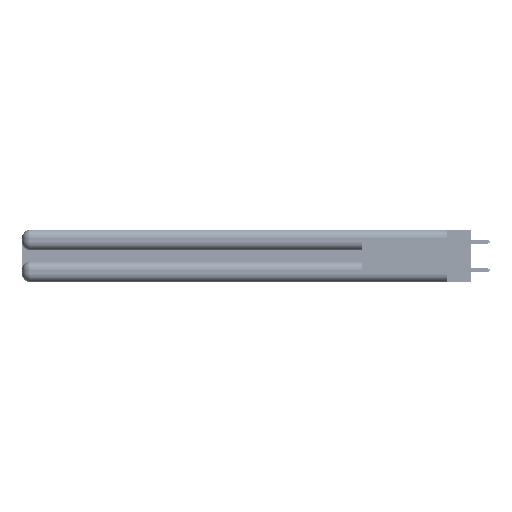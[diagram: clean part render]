
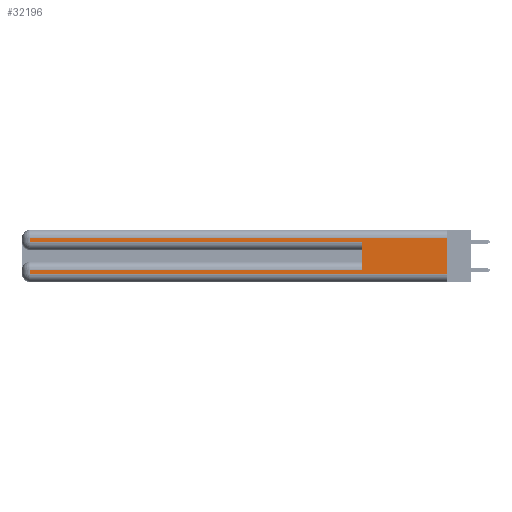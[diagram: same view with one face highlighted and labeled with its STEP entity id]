
A CAD part, left-side view. The second image highlights one B-rep face of the part: STEP entity #32196.
In plain terms, the highlighted planar face has unit normal (-1, 0, 0).
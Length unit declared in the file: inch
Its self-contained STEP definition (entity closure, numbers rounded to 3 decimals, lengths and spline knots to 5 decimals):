
#92 = VERTEX_POINT ( 'NONE', #42001 ) ;
#670 = DIRECTION ( 'NONE',  ( 0., 0., -1. ) ) ;
#1728 = DIRECTION ( 'NONE',  ( 0., 1., 0. ) ) ;
#2706 = EDGE_CURVE ( 'NONE', #34222, #14270, #22295, .T. ) ;
#3669 = CARTESIAN_POINT ( 'NONE',  ( 0., 0., 0.31 ) ) ;
#4077 = CARTESIAN_POINT ( 'NONE',  ( 0., 0., 0.37 ) ) ;
#5230 = VECTOR ( 'NONE', #48398, 39.37008 ) ;
#7872 = ORIENTED_EDGE ( 'NONE', *, *, #2706, .T. ) ;
#8289 = CARTESIAN_POINT ( 'NONE',  ( 0., 2.94, 0.085 ) ) ;
#9274 = DIRECTION ( 'NONE',  ( 0., -1., 0. ) ) ;
#10135 = CARTESIAN_POINT ( 'NONE',  ( 0., 0., 0.31 ) ) ;
#10445 = AXIS2_PLACEMENT_3D ( 'NONE', #50212, #34069, #42154 ) ;
#10638 = VERTEX_POINT ( 'NONE', #8289 ) ;
#11763 = LINE ( 'NONE', #32618, #17405 ) ;
#12158 = VECTOR ( 'NONE', #1728, 39.37008 ) ;
#12441 = VERTEX_POINT ( 'NONE', #10135 ) ;
#12703 = ORIENTED_EDGE ( 'NONE', *, *, #34174, .T. ) ;
#13184 = CARTESIAN_POINT ( 'NONE',  ( 0., 0., 0.06 ) ) ;
#14047 = ORIENTED_EDGE ( 'NONE', *, *, #20607, .F. ) ;
#14270 = VERTEX_POINT ( 'NONE', #13184 ) ;
#14322 = ORIENTED_EDGE ( 'NONE', *, *, #28800, .F. ) ;
#14401 = VECTOR ( 'NONE', #41583, 39.37008 ) ;
#15614 = VERTEX_POINT ( 'NONE', #42710 ) ;
#17405 = VECTOR ( 'NONE', #32457, 39.37008 ) ;
#18414 = LINE ( 'NONE', #4077, #36571 ) ;
#19730 = EDGE_CURVE ( 'NONE', #28810, #15614, #42766, .T. ) ;
#20607 = EDGE_CURVE ( 'NONE', #22252, #92, #23784, .T. ) ;
#21648 = PLANE ( 'NONE',  #10445 ) ;
#21679 = DIRECTION ( 'NONE',  ( 0., 0., 1. ) ) ;
#22252 = VERTEX_POINT ( 'NONE', #28986 ) ;
#22295 = LINE ( 'NONE', #45050, #28575 ) ;
#23784 = LINE ( 'NONE', #49381, #49551 ) ;
#28575 = VECTOR ( 'NONE', #9274, 39.37008 ) ;
#28800 = EDGE_CURVE ( 'NONE', #12441, #14270, #18414, .T. ) ;
#28810 = VERTEX_POINT ( 'NONE', #47279 ) ;
#28986 = CARTESIAN_POINT ( 'NONE',  ( 0., 0.6, 0.085 ) ) ;
#29103 = LINE ( 'NONE', #3669, #5230 ) ;
#29411 = EDGE_LOOP ( 'NONE', ( #14322, #37956, #45199, #12703, #14047, #41851, #46881, #7872 ) ) ;
#31377 = FACE_OUTER_BOUND ( 'NONE', #29411, .T. ) ;
#31816 = DIRECTION ( 'NONE',  ( 0., 0., -1. ) ) ;
#32071 = VECTOR ( 'NONE', #670, 39.37008 ) ;
#32196 = ADVANCED_FACE ( 'NONE', ( #31377 ), #21648, .F. ) ;
#32457 = DIRECTION ( 'NONE',  ( 0., -1., 0. ) ) ;
#32618 = CARTESIAN_POINT ( 'NONE',  ( 0., 0., 0.285 ) ) ;
#33482 = CARTESIAN_POINT ( 'NONE',  ( 0., 2.94, 0.37 ) ) ;
#34069 = DIRECTION ( 'NONE',  ( 1., 0., 0. ) ) ;
#34174 = EDGE_CURVE ( 'NONE', #15614, #92, #11763, .T. ) ;
#34222 = VERTEX_POINT ( 'NONE', #44730 ) ;
#35774 = CARTESIAN_POINT ( 'NONE',  ( 0., 2.94, 0.37 ) ) ;
#36571 = VECTOR ( 'NONE', #31816, 39.37008 ) ;
#37680 = CARTESIAN_POINT ( 'NONE',  ( 0., 0., 0.085 ) ) ;
#37956 = ORIENTED_EDGE ( 'NONE', *, *, #39055, .T. ) ;
#39055 = EDGE_CURVE ( 'NONE', #12441, #28810, #29103, .T. ) ;
#40108 = LINE ( 'NONE', #33482, #14401 ) ;
#41583 = DIRECTION ( 'NONE',  ( 0., 0., -1. ) ) ;
#41851 = ORIENTED_EDGE ( 'NONE', *, *, #45974, .T. ) ;
#42001 = CARTESIAN_POINT ( 'NONE',  ( 0., 0.6, 0.285 ) ) ;
#42154 = DIRECTION ( 'NONE',  ( 0., 0., -1. ) ) ;
#42710 = CARTESIAN_POINT ( 'NONE',  ( 0., 2.94, 0.285 ) ) ;
#42766 = LINE ( 'NONE', #35774, #32071 ) ;
#42927 = LINE ( 'NONE', #37680, #12158 ) ;
#44730 = CARTESIAN_POINT ( 'NONE',  ( 0., 2.94, 0.06 ) ) ;
#45050 = CARTESIAN_POINT ( 'NONE',  ( 0., 0., 0.06 ) ) ;
#45199 = ORIENTED_EDGE ( 'NONE', *, *, #19730, .T. ) ;
#45974 = EDGE_CURVE ( 'NONE', #22252, #10638, #42927, .T. ) ;
#46881 = ORIENTED_EDGE ( 'NONE', *, *, #49255, .T. ) ;
#47279 = CARTESIAN_POINT ( 'NONE',  ( 0., 2.94, 0.31 ) ) ;
#48398 = DIRECTION ( 'NONE',  ( 0., 1., 0. ) ) ;
#49255 = EDGE_CURVE ( 'NONE', #10638, #34222, #40108, .T. ) ;
#49381 = CARTESIAN_POINT ( 'NONE',  ( 0., 0.6, 0.145 ) ) ;
#49551 = VECTOR ( 'NONE', #21679, 39.37008 ) ;
#50212 = CARTESIAN_POINT ( 'NONE',  ( 0., 0., 0.37 ) ) ;
